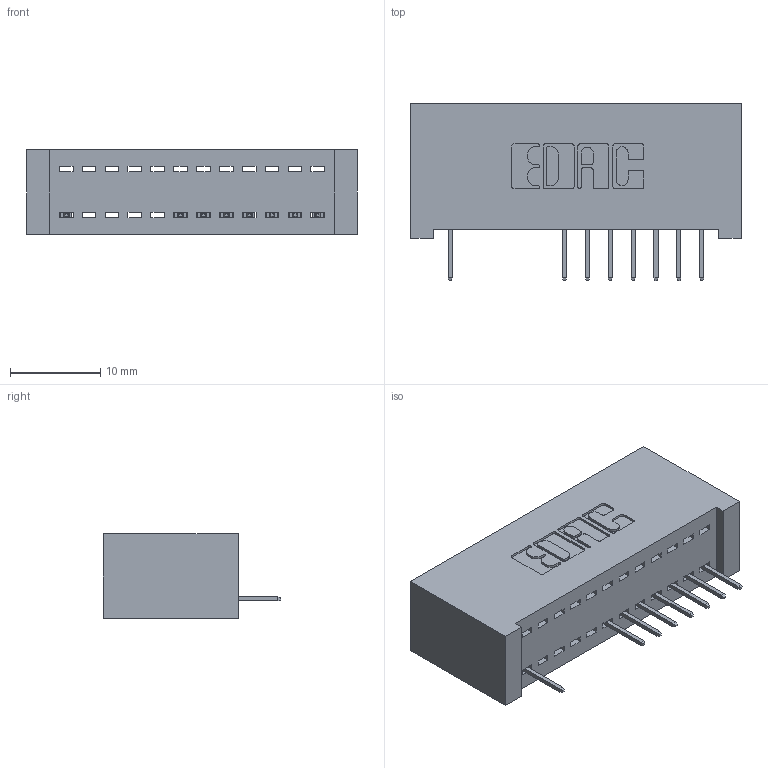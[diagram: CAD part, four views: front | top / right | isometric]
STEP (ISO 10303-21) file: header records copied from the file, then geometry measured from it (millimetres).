
FILE_DESCRIPTION (( 'STEP AP203' ), '1' );
FILE_NAME ('392-012-524-101.STEP', '2018-08-14T21:54:40', ( '' ), ( '' ), 'SwSTEP 2.0', 'SolidWorks 2016', '' );
FILE_SCHEMA (( 'CONFIG_CONTROL_DESIGN' ));
Length unit declared in the file: inch
Products named in the file (3): 342 Part_Lugless; 345-292-001_345-293-124; 392-012-524-101
Assembly tree (9 placements, depth 2):
  392-012-524-101
    342 Part_Lugless
    345-292-001_345-293-124  x8
Bounding box: 36.73 x 19.69 x 9.4 mm (x, y, z)
Volume: 3441.5 mm3; surface area: 4481.6 mm2
Topology: 9 solids, 9 shells, 646 faces, 1883 edges, 1222 vertices
Faces by surface type: plane 494, cylinder 152
Entity records: 10753 total; most frequent: CARTESIAN_POINT 1882, ORIENTED_EDGE 1834, DIRECTION 1637, EDGE_CURVE 917, LINE 801, VECTOR 801, VERTEX_POINT 606, AXIS2_PLACEMENT_3D 418
